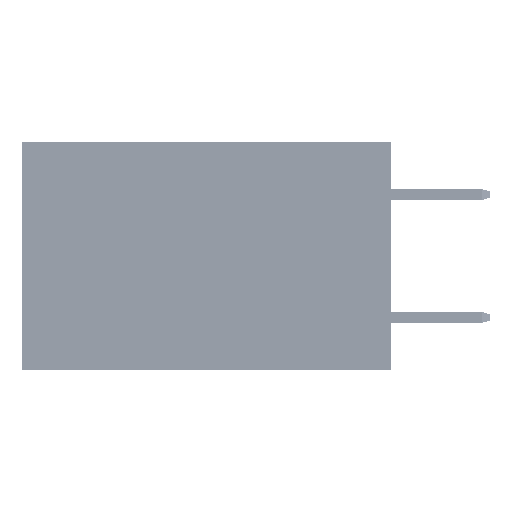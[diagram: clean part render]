
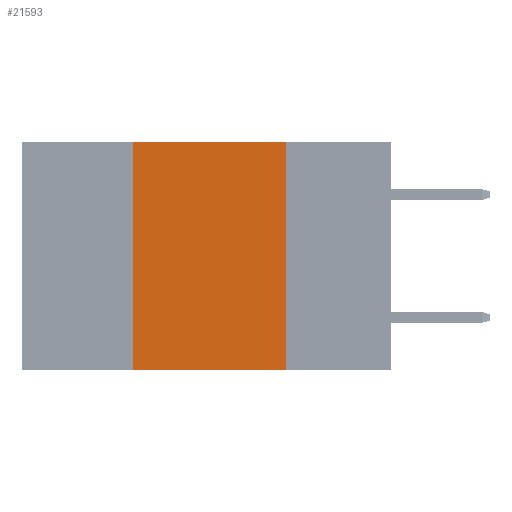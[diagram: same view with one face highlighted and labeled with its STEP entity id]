
A CAD part, left-side view. The second image highlights one B-rep face of the part: STEP entity #21593.
In plain terms, the highlighted planar face has unit normal (-1, 0, 0).
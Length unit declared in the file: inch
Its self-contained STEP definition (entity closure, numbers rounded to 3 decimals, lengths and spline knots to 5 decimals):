
#93 = ORIENTED_EDGE ( 'NONE', *, *, #34017, .T. ) ;
#1800 = CARTESIAN_POINT ( 'NONE',  ( 0., 0.6, 0. ) ) ;
#2500 = PLANE ( 'NONE',  #34853 ) ;
#4896 = CARTESIAN_POINT ( 'NONE',  ( 0., 0.17, 0. ) ) ;
#8026 = VECTOR ( 'NONE', #48857, 39.37008 ) ;
#8087 = VERTEX_POINT ( 'NONE', #37489 ) ;
#9039 = VERTEX_POINT ( 'NONE', #26622 ) ;
#9246 = CARTESIAN_POINT ( 'NONE',  ( 0., 0.17, 0. ) ) ;
#11902 = LINE ( 'NONE', #36467, #8026 ) ;
#12040 = FACE_OUTER_BOUND ( 'NONE', #26394, .T. ) ;
#17846 = ORIENTED_EDGE ( 'NONE', *, *, #41270, .F. ) ;
#18078 = LINE ( 'NONE', #31002, #29774 ) ;
#18863 = EDGE_CURVE ( 'NONE', #8087, #51748, #11902, .T. ) ;
#21593 = ADVANCED_FACE ( 'NONE', ( #12040 ), #2500, .F. ) ;
#24636 = LINE ( 'NONE', #49986, #29854 ) ;
#25401 = VECTOR ( 'NONE', #33939, 39.37008 ) ;
#26342 = ORIENTED_EDGE ( 'NONE', *, *, #45201, .F. ) ;
#26394 = EDGE_LOOP ( 'NONE', ( #26342, #41806, #17846, #93 ) ) ;
#26622 = CARTESIAN_POINT ( 'NONE',  ( 0., 0.17, -0.37 ) ) ;
#29774 = VECTOR ( 'NONE', #43251, 39.37008 ) ;
#29854 = VECTOR ( 'NONE', #32849, 39.37008 ) ;
#30608 = LINE ( 'NONE', #4896, #25401 ) ;
#31002 = CARTESIAN_POINT ( 'NONE',  ( 0., 0.42, 0. ) ) ;
#32849 = DIRECTION ( 'NONE',  ( 0., -1., 0. ) ) ;
#33939 = DIRECTION ( 'NONE',  ( 0., 0., -1. ) ) ;
#34017 = EDGE_CURVE ( 'NONE', #46643, #9039, #24636, .T. ) ;
#34853 = AXIS2_PLACEMENT_3D ( 'NONE', #1800, #43775, #47620 ) ;
#36467 = CARTESIAN_POINT ( 'NONE',  ( 0., 0.6, 0. ) ) ;
#37489 = CARTESIAN_POINT ( 'NONE',  ( 0., 0.42, 0. ) ) ;
#41270 = EDGE_CURVE ( 'NONE', #46643, #8087, #18078, .T. ) ;
#41806 = ORIENTED_EDGE ( 'NONE', *, *, #18863, .F. ) ;
#43251 = DIRECTION ( 'NONE',  ( 0., 0., 1. ) ) ;
#43775 = DIRECTION ( 'NONE',  ( 1., 0., 0. ) ) ;
#45201 = EDGE_CURVE ( 'NONE', #51748, #9039, #30608, .T. ) ;
#45285 = CARTESIAN_POINT ( 'NONE',  ( 0., 0.42, -0.37 ) ) ;
#46643 = VERTEX_POINT ( 'NONE', #45285 ) ;
#47620 = DIRECTION ( 'NONE',  ( 0., 0., -1. ) ) ;
#48857 = DIRECTION ( 'NONE',  ( 0., -1., 0. ) ) ;
#49986 = CARTESIAN_POINT ( 'NONE',  ( 0., 0.6, -0.37 ) ) ;
#51748 = VERTEX_POINT ( 'NONE', #9246 ) ;
